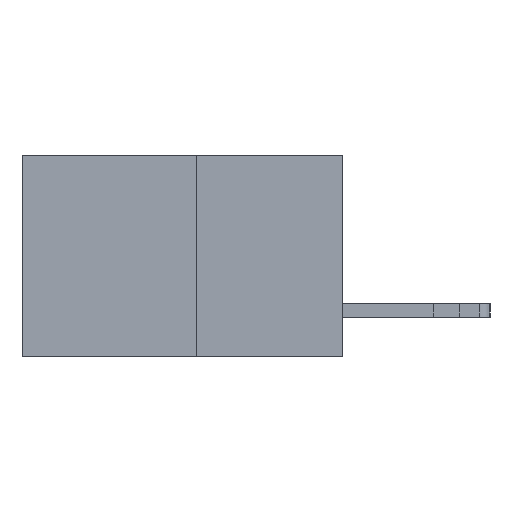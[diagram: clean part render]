
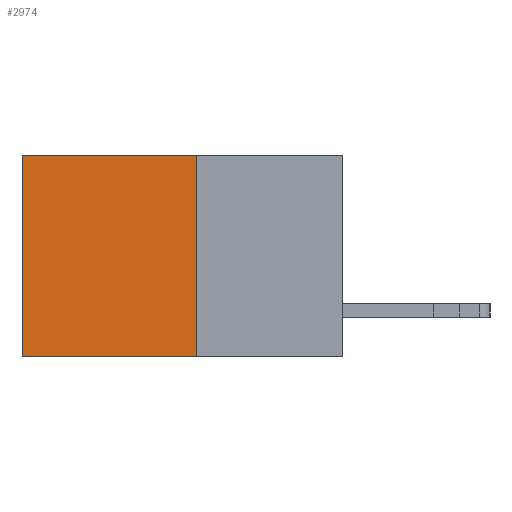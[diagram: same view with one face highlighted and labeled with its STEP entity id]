
A CAD part, left-side view. The second image highlights one B-rep face of the part: STEP entity #2974.
In plain terms, the highlighted planar face has unit normal (-1, 0, 0).
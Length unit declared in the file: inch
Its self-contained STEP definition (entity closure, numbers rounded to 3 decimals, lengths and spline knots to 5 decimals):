
#533 = EDGE_CURVE ( 'NONE', #3255, #8528, #3232, .T. ) ;
#864 = VERTEX_POINT ( 'NONE', #7451 ) ;
#1148 = ORIENTED_EDGE ( 'NONE', *, *, #10886, .F. ) ;
#1538 = DIRECTION ( 'NONE',  ( 0., 0., -1. ) ) ;
#1803 = DIRECTION ( 'NONE',  ( 1., 0., 0. ) ) ;
#1912 = CARTESIAN_POINT ( 'NONE',  ( 0.277, 0.59, -0.37 ) ) ;
#2001 = VECTOR ( 'NONE', #3173, 39.37008 ) ;
#2127 = CARTESIAN_POINT ( 'NONE',  ( 0.277, 0.27, -0.37 ) ) ;
#2414 = CARTESIAN_POINT ( 'NONE',  ( 0.277, 0.27, 0. ) ) ;
#2974 = ADVANCED_FACE ( 'NONE', ( #13274 ), #11118, .F. ) ;
#3173 = DIRECTION ( 'NONE',  ( 0., 0., -1. ) ) ;
#3232 = LINE ( 'NONE', #2414, #11374 ) ;
#3255 = VERTEX_POINT ( 'NONE', #11037 ) ;
#4424 = DIRECTION ( 'NONE',  ( 0., 0., -1. ) ) ;
#5071 = VERTEX_POINT ( 'NONE', #1912 ) ;
#5590 = VECTOR ( 'NONE', #4424, 39.37008 ) ;
#5629 = CARTESIAN_POINT ( 'NONE',  ( 0.277, 0.59, 0. ) ) ;
#5895 = LINE ( 'NONE', #11813, #5590 ) ;
#6824 = CARTESIAN_POINT ( 'NONE',  ( 0.277, 0.27, -0.37 ) ) ;
#7276 = VECTOR ( 'NONE', #10805, 39.37008 ) ;
#7374 = DIRECTION ( 'NONE',  ( 0., 1., 0. ) ) ;
#7451 = CARTESIAN_POINT ( 'NONE',  ( 0.277, 0.27, -0.37 ) ) ;
#7752 = EDGE_LOOP ( 'NONE', ( #11062, #12003, #1148, #9589 ) ) ;
#8130 = EDGE_CURVE ( 'NONE', #864, #5071, #9877, .T. ) ;
#8528 = VERTEX_POINT ( 'NONE', #5629 ) ;
#9372 = CARTESIAN_POINT ( 'NONE',  ( 0.277, 0.27, -0.37 ) ) ;
#9589 = ORIENTED_EDGE ( 'NONE', *, *, #533, .T. ) ;
#9877 = LINE ( 'NONE', #9372, #7276 ) ;
#10466 = LINE ( 'NONE', #2127, #2001 ) ;
#10805 = DIRECTION ( 'NONE',  ( 0., 1., 0. ) ) ;
#10886 = EDGE_CURVE ( 'NONE', #3255, #864, #10466, .T. ) ;
#11029 = EDGE_CURVE ( 'NONE', #8528, #5071, #5895, .T. ) ;
#11037 = CARTESIAN_POINT ( 'NONE',  ( 0.277, 0.27, 0. ) ) ;
#11062 = ORIENTED_EDGE ( 'NONE', *, *, #11029, .T. ) ;
#11118 = PLANE ( 'NONE',  #11323 ) ;
#11323 = AXIS2_PLACEMENT_3D ( 'NONE', #6824, #1803, #1538 ) ;
#11374 = VECTOR ( 'NONE', #7374, 39.37008 ) ;
#11813 = CARTESIAN_POINT ( 'NONE',  ( 0.277, 0.59, -0.37 ) ) ;
#12003 = ORIENTED_EDGE ( 'NONE', *, *, #8130, .F. ) ;
#13274 = FACE_OUTER_BOUND ( 'NONE', #7752, .T. ) ;
